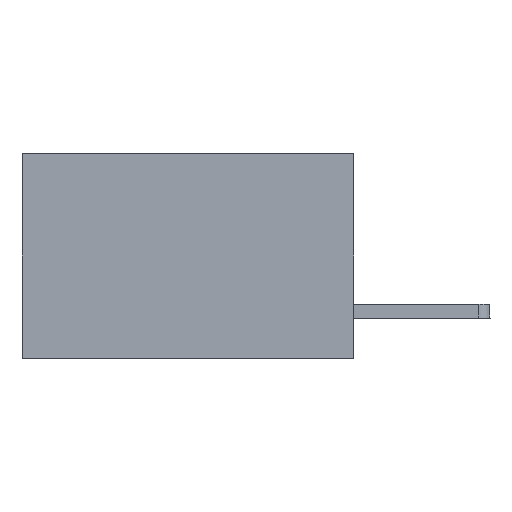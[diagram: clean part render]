
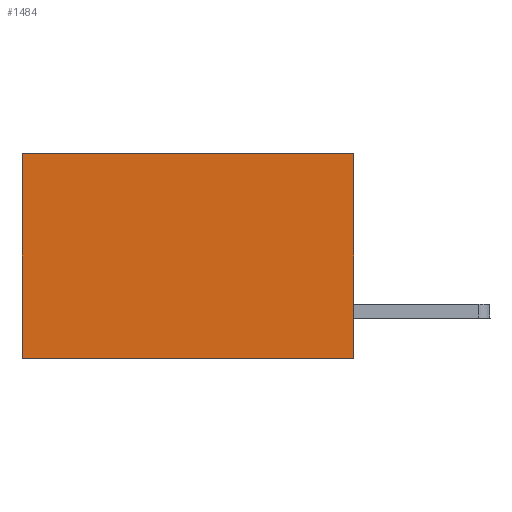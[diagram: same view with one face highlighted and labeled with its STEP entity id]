
A CAD part, left-side view. The second image highlights one B-rep face of the part: STEP entity #1484.
In plain terms, the highlighted planar face has unit normal (-1, 0, 0).
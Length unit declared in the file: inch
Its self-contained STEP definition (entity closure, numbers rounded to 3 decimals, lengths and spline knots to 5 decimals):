
#855 = VECTOR ( 'NONE', #6685, 39.37008 ) ;
#1484 = ADVANCED_FACE ( 'NONE', ( #9331 ), #8114, .F. ) ;
#1530 = DIRECTION ( 'NONE',  ( 0., 1., 0. ) ) ;
#2419 = ORIENTED_EDGE ( 'NONE', *, *, #5322, .T. ) ;
#2657 = CARTESIAN_POINT ( 'NONE',  ( 0.2875, 0., -0.37 ) ) ;
#3201 = CARTESIAN_POINT ( 'NONE',  ( 0.2875, 0., 0. ) ) ;
#3302 = VECTOR ( 'NONE', #1530, 39.37008 ) ;
#3757 = LINE ( 'NONE', #7665, #855 ) ;
#3832 = LINE ( 'NONE', #7874, #4930 ) ;
#3964 = EDGE_CURVE ( 'NONE', #9301, #6159, #3832, .T. ) ;
#4248 = ORIENTED_EDGE ( 'NONE', *, *, #12723, .T. ) ;
#4930 = VECTOR ( 'NONE', #9873, 39.37008 ) ;
#5322 = EDGE_CURVE ( 'NONE', #12225, #7618, #3757, .T. ) ;
#5901 = VECTOR ( 'NONE', #7636, 39.37008 ) ;
#6159 = VERTEX_POINT ( 'NONE', #8810 ) ;
#6685 = DIRECTION ( 'NONE',  ( 0., 0., -1. ) ) ;
#7385 = ORIENTED_EDGE ( 'NONE', *, *, #3964, .F. ) ;
#7386 = CARTESIAN_POINT ( 'NONE',  ( 0.2875, 0., 0. ) ) ;
#7507 = CARTESIAN_POINT ( 'NONE',  ( 0.2875, 0.6, 0. ) ) ;
#7618 = VERTEX_POINT ( 'NONE', #10408 ) ;
#7636 = DIRECTION ( 'NONE',  ( 0., 1., 0. ) ) ;
#7665 = CARTESIAN_POINT ( 'NONE',  ( 0.2875, 0.6, 0. ) ) ;
#7874 = CARTESIAN_POINT ( 'NONE',  ( 0.2875, 0., 0. ) ) ;
#8105 = EDGE_LOOP ( 'NONE', ( #2419, #9125, #7385, #4248 ) ) ;
#8114 = PLANE ( 'NONE',  #8305 ) ;
#8210 = DIRECTION ( 'NONE',  ( 1., 0., 0. ) ) ;
#8305 = AXIS2_PLACEMENT_3D ( 'NONE', #3201, #8210, #11120 ) ;
#8537 = LINE ( 'NONE', #7386, #5901 ) ;
#8810 = CARTESIAN_POINT ( 'NONE',  ( 0.2875, 0., -0.37 ) ) ;
#9125 = ORIENTED_EDGE ( 'NONE', *, *, #11041, .F. ) ;
#9301 = VERTEX_POINT ( 'NONE', #9930 ) ;
#9331 = FACE_OUTER_BOUND ( 'NONE', #8105, .T. ) ;
#9873 = DIRECTION ( 'NONE',  ( 0., 0., -1. ) ) ;
#9930 = CARTESIAN_POINT ( 'NONE',  ( 0.2875, 0., 0. ) ) ;
#10070 = LINE ( 'NONE', #2657, #3302 ) ;
#10408 = CARTESIAN_POINT ( 'NONE',  ( 0.2875, 0.6, -0.37 ) ) ;
#11041 = EDGE_CURVE ( 'NONE', #6159, #7618, #10070, .T. ) ;
#11120 = DIRECTION ( 'NONE',  ( 0., 0., -1. ) ) ;
#12225 = VERTEX_POINT ( 'NONE', #7507 ) ;
#12723 = EDGE_CURVE ( 'NONE', #9301, #12225, #8537, .T. ) ;
